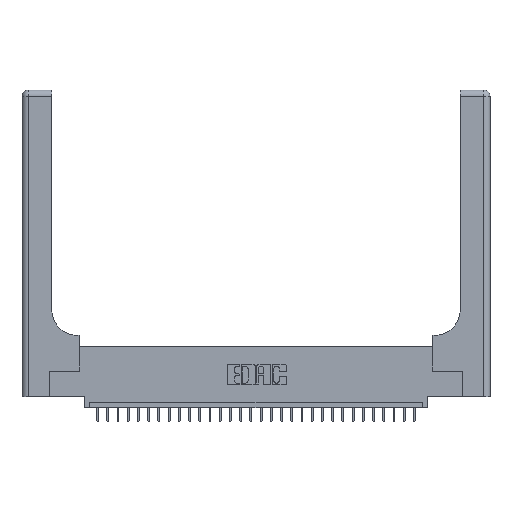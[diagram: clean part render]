
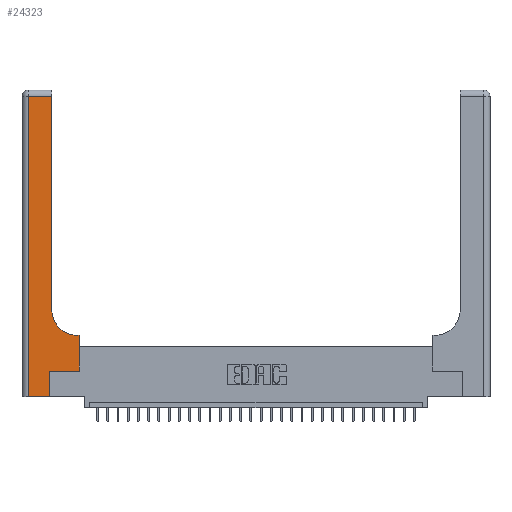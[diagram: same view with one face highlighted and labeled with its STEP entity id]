
A CAD part, top view. The second image highlights one B-rep face of the part: STEP entity #24323.
In plain terms, the highlighted planar face has unit normal (0, 0, 1).
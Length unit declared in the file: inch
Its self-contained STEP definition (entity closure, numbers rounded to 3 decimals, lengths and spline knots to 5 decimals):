
#236 = ORIENTED_EDGE ( 'NONE', *, *, #2373, .T. ) ;
#423 = LINE ( 'NONE', #6286, #10236 ) ;
#526 = CARTESIAN_POINT ( 'NONE',  ( 0., 3., 0.37 ) ) ;
#751 = ORIENTED_EDGE ( 'NONE', *, *, #30538, .T. ) ;
#1221 = VERTEX_POINT ( 'NONE', #26586 ) ;
#1410 = CARTESIAN_POINT ( 'NONE',  ( 0.06, 3., 0.37 ) ) ;
#2302 = CARTESIAN_POINT ( 'NONE',  ( 0.5415, 0.85, 0.37 ) ) ;
#2347 = EDGE_CURVE ( 'NONE', #1221, #14134, #11040, .T. ) ;
#2373 = EDGE_CURVE ( 'NONE', #3838, #11926, #28053, .T. ) ;
#2556 = EDGE_CURVE ( 'NONE', #7789, #27679, #423, .T. ) ;
#3156 = DIRECTION ( 'NONE',  ( -1., 0., 0. ) ) ;
#3305 = CARTESIAN_POINT ( 'NONE',  ( 0., 2.94, 0.37 ) ) ;
#3838 = VERTEX_POINT ( 'NONE', #22870 ) ;
#3883 = DIRECTION ( 'NONE',  ( 0., 1., 0. ) ) ;
#4366 = CARTESIAN_POINT ( 'NONE',  ( 0.269, 0.25, 0.37 ) ) ;
#4592 = CARTESIAN_POINT ( 'NONE',  ( 0.269, 0.25, 0.37 ) ) ;
#4724 = LINE ( 'NONE', #28416, #12994 ) ;
#4868 = AXIS2_PLACEMENT_3D ( 'NONE', #526, #26428, #5067 ) ;
#4961 = DIRECTION ( 'NONE',  ( 0., 0., -1. ) ) ;
#5067 = DIRECTION ( 'NONE',  ( -1., 0., 0. ) ) ;
#5618 = CARTESIAN_POINT ( 'NONE',  ( 0.5585, 0.6, 0.37 ) ) ;
#5677 = ORIENTED_EDGE ( 'NONE', *, *, #5953, .T. ) ;
#5953 = EDGE_CURVE ( 'NONE', #22240, #7789, #4724, .T. ) ;
#6286 = CARTESIAN_POINT ( 'NONE',  ( 0.269, 0., 0.37 ) ) ;
#6675 = CARTESIAN_POINT ( 'NONE',  ( 0.2915, 3., 0.37 ) ) ;
#7789 = VERTEX_POINT ( 'NONE', #14083 ) ;
#8412 = EDGE_CURVE ( 'NONE', #11926, #19394, #24531, .T. ) ;
#9054 = LINE ( 'NONE', #1410, #12416 ) ;
#10236 = VECTOR ( 'NONE', #29117, 39.37008 ) ;
#10500 = CARTESIAN_POINT ( 'NONE',  ( 0.5415, 0.6, 0.37 ) ) ;
#11040 = LINE ( 'NONE', #20402, #14726 ) ;
#11280 = AXIS2_PLACEMENT_3D ( 'NONE', #2302, #4961, #11965 ) ;
#11911 = ORIENTED_EDGE ( 'NONE', *, *, #8412, .T. ) ;
#11922 = VECTOR ( 'NONE', #20875, 39.37008 ) ;
#11926 = VERTEX_POINT ( 'NONE', #19813 ) ;
#11965 = DIRECTION ( 'NONE',  ( 1., 0., 0. ) ) ;
#12225 = VECTOR ( 'NONE', #3883, 39.37008 ) ;
#12416 = VECTOR ( 'NONE', #13278, 39.37008 ) ;
#12731 = CARTESIAN_POINT ( 'NONE',  ( 0.06, 0., 0.37 ) ) ;
#12994 = VECTOR ( 'NONE', #22851, 39.37008 ) ;
#13027 = ORIENTED_EDGE ( 'NONE', *, *, #28112, .T. ) ;
#13278 = DIRECTION ( 'NONE',  ( 0., -1., 0. ) ) ;
#13390 = CARTESIAN_POINT ( 'NONE',  ( 0.2915, 0.6, 0.37 ) ) ;
#14083 = CARTESIAN_POINT ( 'NONE',  ( 0.269, 0., 0.37 ) ) ;
#14134 = VERTEX_POINT ( 'NONE', #5618 ) ;
#14584 = PLANE ( 'NONE',  #4868 ) ;
#14726 = VECTOR ( 'NONE', #16043, 39.37008 ) ;
#16043 = DIRECTION ( 'NONE',  ( 0., 1., 0. ) ) ;
#16740 = DIRECTION ( 'NONE',  ( 1., 0., 0. ) ) ;
#16867 = CARTESIAN_POINT ( 'NONE',  ( 0.06, 2.94, 0.37 ) ) ;
#17983 = VECTOR ( 'NONE', #16740, 39.37008 ) ;
#19394 = VERTEX_POINT ( 'NONE', #16867 ) ;
#19705 = FACE_OUTER_BOUND ( 'NONE', #25619, .T. ) ;
#19813 = CARTESIAN_POINT ( 'NONE',  ( 0.2915, 2.94, 0.37 ) ) ;
#20402 = CARTESIAN_POINT ( 'NONE',  ( 0.5585, 0.25, 0.37 ) ) ;
#20441 = ORIENTED_EDGE ( 'NONE', *, *, #2556, .T. ) ;
#20565 = LINE ( 'NONE', #13390, #11922 ) ;
#20804 = LINE ( 'NONE', #4592, #17983 ) ;
#20875 = DIRECTION ( 'NONE',  ( -1., 0., 0. ) ) ;
#22228 = ORIENTED_EDGE ( 'NONE', *, *, #2347, .T. ) ;
#22240 = VERTEX_POINT ( 'NONE', #12731 ) ;
#22851 = DIRECTION ( 'NONE',  ( 1., 0., 0. ) ) ;
#22870 = CARTESIAN_POINT ( 'NONE',  ( 0.2915, 0.85, 0.37 ) ) ;
#23329 = EDGE_CURVE ( 'NONE', #26634, #3838, #28234, .T. ) ;
#24323 = ADVANCED_FACE ( 'NONE', ( #19705 ), #14584, .F. ) ;
#24407 = ORIENTED_EDGE ( 'NONE', *, *, #28543, .T. ) ;
#24531 = LINE ( 'NONE', #3305, #25349 ) ;
#25349 = VECTOR ( 'NONE', #3156, 39.37008 ) ;
#25619 = EDGE_LOOP ( 'NONE', ( #236, #11911, #13027, #5677, #20441, #751, #22228, #24407, #28556 ) ) ;
#26428 = DIRECTION ( 'NONE',  ( 0., 0., -1. ) ) ;
#26586 = CARTESIAN_POINT ( 'NONE',  ( 0.5585, 0.25, 0.37 ) ) ;
#26634 = VERTEX_POINT ( 'NONE', #10500 ) ;
#27679 = VERTEX_POINT ( 'NONE', #4366 ) ;
#28053 = LINE ( 'NONE', #6675, #12225 ) ;
#28112 = EDGE_CURVE ( 'NONE', #19394, #22240, #9054, .T. ) ;
#28234 = CIRCLE ( 'NONE', #11280, 0.25 ) ;
#28416 = CARTESIAN_POINT ( 'NONE',  ( 0., 0., 0.37 ) ) ;
#28543 = EDGE_CURVE ( 'NONE', #14134, #26634, #20565, .T. ) ;
#28556 = ORIENTED_EDGE ( 'NONE', *, *, #23329, .T. ) ;
#29117 = DIRECTION ( 'NONE',  ( 0., 1., 0. ) ) ;
#30538 = EDGE_CURVE ( 'NONE', #27679, #1221, #20804, .T. ) ;
